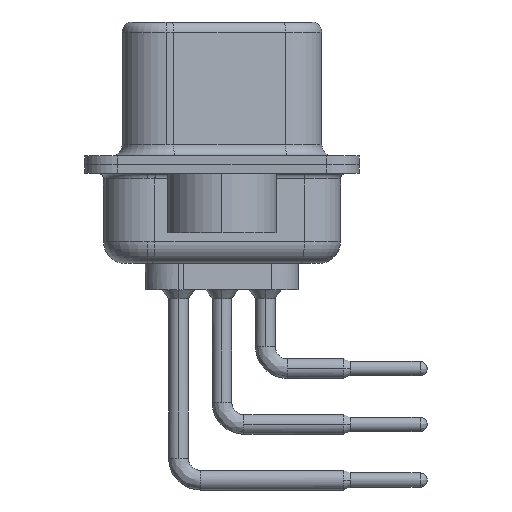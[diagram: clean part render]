
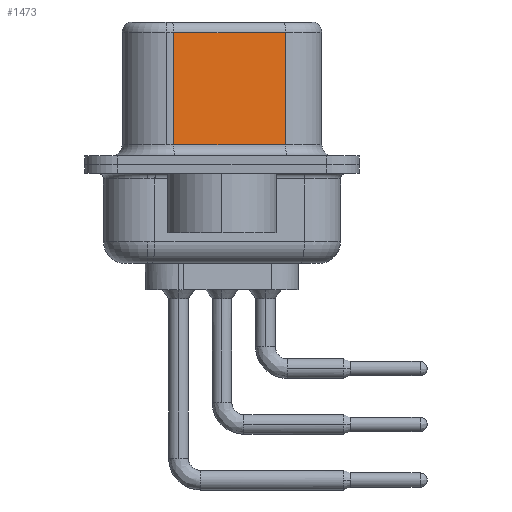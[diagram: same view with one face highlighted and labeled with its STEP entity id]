
A CAD part, left-side view. The second image highlights one B-rep face of the part: STEP entity #1473.
In plain terms, the highlighted planar face has unit normal (-0.985, -0.174, 0).
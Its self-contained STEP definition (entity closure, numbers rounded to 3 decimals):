
#1473 = ADVANCED_FACE ( 'NONE', ( #3187 ), #4707, .F. ) ;
#3151 = DIRECTION ( 'NONE',  ( 0., 0., -1. ) ) ;
#3187 = FACE_OUTER_BOUND ( 'NONE', #29903, .T. ) ;
#4216 = CARTESIAN_POINT ( 'NONE',  ( 3.68, 2.203, 6.52 ) ) ;
#4707 = PLANE ( 'NONE',  #31482 ) ;
#5830 = CARTESIAN_POINT ( 'NONE',  ( 4.58, -2.897, 6.52 ) ) ;
#6427 = LINE ( 'NONE', #27306, #12720 ) ;
#7265 = ORIENTED_EDGE ( 'NONE', *, *, #22782, .T. ) ;
#7885 = ORIENTED_EDGE ( 'NONE', *, *, #25164, .T. ) ;
#8169 = VECTOR ( 'NONE', #12282, 1000. ) ;
#8619 = LINE ( 'NONE', #5830, #29019 ) ;
#9582 = CARTESIAN_POINT ( 'NONE',  ( 4.58, -2.897, 0.9 ) ) ;
#10679 = LINE ( 'NONE', #9582, #31053 ) ;
#12282 = DIRECTION ( 'NONE',  ( 0., 0., -1. ) ) ;
#12720 = VECTOR ( 'NONE', #29988, 1000. ) ;
#12878 = DIRECTION ( 'NONE',  ( -0.174, 0.985, 0. ) ) ;
#12964 = DIRECTION ( 'NONE',  ( 0.985, 0.174, 0. ) ) ;
#14850 = CARTESIAN_POINT ( 'NONE',  ( 3.68, 2.203, 6.02 ) ) ;
#15587 = VERTEX_POINT ( 'NONE', #28135 ) ;
#16079 = LINE ( 'NONE', #4216, #8169 ) ;
#18766 = CARTESIAN_POINT ( 'NONE',  ( 4.58, -2.897, 6.02 ) ) ;
#20559 = CARTESIAN_POINT ( 'NONE',  ( 3.68, 2.203, 0.9 ) ) ;
#22782 = EDGE_CURVE ( 'NONE', #27408, #23462, #16079, .T. ) ;
#23462 = VERTEX_POINT ( 'NONE', #20559 ) ;
#25164 = EDGE_CURVE ( 'NONE', #27068, #27408, #6427, .T. ) ;
#27068 = VERTEX_POINT ( 'NONE', #18766 ) ;
#27306 = CARTESIAN_POINT ( 'NONE',  ( 4.58, -2.897, 6.02 ) ) ;
#27408 = VERTEX_POINT ( 'NONE', #14850 ) ;
#28053 = DIRECTION ( 'NONE',  ( 0.174, -0.985, 0. ) ) ;
#28135 = CARTESIAN_POINT ( 'NONE',  ( 4.58, -2.897, 0.9 ) ) ;
#29019 = VECTOR ( 'NONE', #3151, 1000. ) ;
#29176 = ORIENTED_EDGE ( 'NONE', *, *, #31900, .F. ) ;
#29903 = EDGE_LOOP ( 'NONE', ( #29176, #7885, #7265, #31979 ) ) ;
#29988 = DIRECTION ( 'NONE',  ( -0.174, 0.985, 0. ) ) ;
#31053 = VECTOR ( 'NONE', #28053, 1000. ) ;
#31328 = CARTESIAN_POINT ( 'NONE',  ( 4.58, -2.897, 6.52 ) ) ;
#31482 = AXIS2_PLACEMENT_3D ( 'NONE', #31328, #12964, #12878 ) ;
#31900 = EDGE_CURVE ( 'NONE', #27068, #15587, #8619, .T. ) ;
#31979 = ORIENTED_EDGE ( 'NONE', *, *, #32604, .T. ) ;
#32604 = EDGE_CURVE ( 'NONE', #23462, #15587, #10679, .T. ) ;
